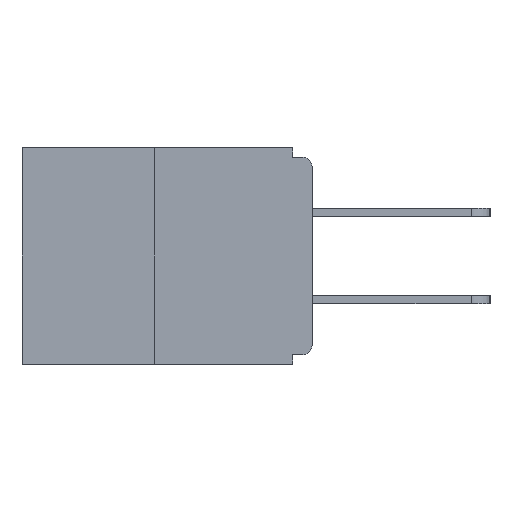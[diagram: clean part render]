
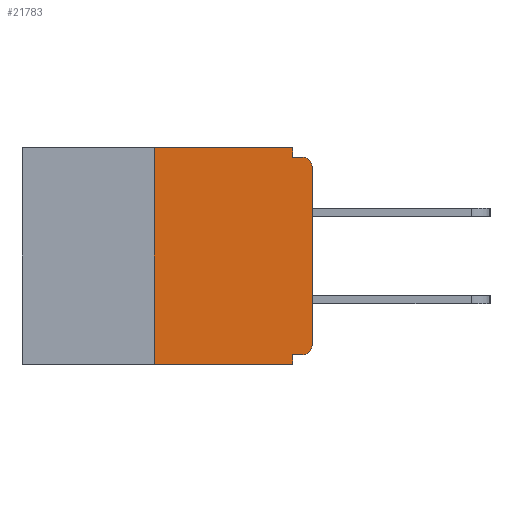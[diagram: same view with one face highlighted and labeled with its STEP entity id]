
A CAD part, left-side view. The second image highlights one B-rep face of the part: STEP entity #21783.
In plain terms, the highlighted planar face has unit normal (-1, 0, 0).
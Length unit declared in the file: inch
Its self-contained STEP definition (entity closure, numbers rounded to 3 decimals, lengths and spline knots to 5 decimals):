
#169 = EDGE_CURVE ( 'NONE', #12513, #19500, #6152, .T. ) ;
#231 = EDGE_CURVE ( 'NONE', #21958, #9194, #2474, .T. ) ;
#364 = DIRECTION ( 'NONE',  ( 0., 0., -1. ) ) ;
#468 = ORIENTED_EDGE ( 'NONE', *, *, #21047, .T. ) ;
#714 = EDGE_CURVE ( 'NONE', #6927, #9710, #7047, .T. ) ;
#760 = VERTEX_POINT ( 'NONE', #4860 ) ;
#1983 = VECTOR ( 'NONE', #9508, 39.37008 ) ;
#2123 = DIRECTION ( 'NONE',  ( 0., 1., 0. ) ) ;
#2136 = VECTOR ( 'NONE', #15917, 39.37008 ) ;
#2330 = EDGE_CURVE ( 'NONE', #12513, #8698, #7003, .T. ) ;
#2474 = LINE ( 'NONE', #5715, #12656 ) ;
#2747 = LINE ( 'NONE', #5709, #2136 ) ;
#3115 = LINE ( 'NONE', #14092, #24157 ) ;
#3269 = VECTOR ( 'NONE', #8938, 39.37008 ) ;
#3313 = PLANE ( 'NONE',  #25467 ) ;
#4295 = CARTESIAN_POINT ( 'NONE',  ( 0., 0.015, -0.03 ) ) ;
#4860 = CARTESIAN_POINT ( 'NONE',  ( 0., 0., -0.313 ) ) ;
#4899 = VECTOR ( 'NONE', #12804, 39.37008 ) ;
#5003 = ORIENTED_EDGE ( 'NONE', *, *, #16083, .T. ) ;
#5268 = CARTESIAN_POINT ( 'NONE',  ( 0., 0.015, -0.313 ) ) ;
#5463 = DIRECTION ( 'NONE',  ( 1., 0., 0. ) ) ;
#5709 = CARTESIAN_POINT ( 'NONE',  ( 0., 0., 0. ) ) ;
#5710 = ORIENTED_EDGE ( 'NONE', *, *, #19974, .T. ) ;
#5715 = CARTESIAN_POINT ( 'NONE',  ( 0., 0., -0.328 ) ) ;
#5799 = CARTESIAN_POINT ( 'NONE',  ( 0., 0.25, 0. ) ) ;
#5900 = ORIENTED_EDGE ( 'NONE', *, *, #2330, .T. ) ;
#6152 = LINE ( 'NONE', #5799, #16676 ) ;
#6377 = EDGE_CURVE ( 'NONE', #19500, #6927, #15220, .T. ) ;
#6667 = CARTESIAN_POINT ( 'NONE',  ( 0., 0.031, 0. ) ) ;
#6927 = VERTEX_POINT ( 'NONE', #13416 ) ;
#7003 = LINE ( 'NONE', #14622, #3269 ) ;
#7047 = LINE ( 'NONE', #6667, #4899 ) ;
#7219 = LINE ( 'NONE', #25058, #1983 ) ;
#8148 = VECTOR ( 'NONE', #19521, 39.37008 ) ;
#8647 = DIRECTION ( 'NONE',  ( 0., 0., -1. ) ) ;
#8698 = VERTEX_POINT ( 'NONE', #9263 ) ;
#8938 = DIRECTION ( 'NONE',  ( 0., -1., 0. ) ) ;
#9194 = VERTEX_POINT ( 'NONE', #22980 ) ;
#9197 = CARTESIAN_POINT ( 'NONE',  ( 0., 0., -0.03 ) ) ;
#9263 = CARTESIAN_POINT ( 'NONE',  ( 0., 0.031, -0.343 ) ) ;
#9508 = DIRECTION ( 'NONE',  ( 0., -1., 0. ) ) ;
#9710 = VERTEX_POINT ( 'NONE', #12374 ) ;
#10007 = DIRECTION ( 'NONE',  ( -1., 0., 0. ) ) ;
#10283 = ORIENTED_EDGE ( 'NONE', *, *, #24113, .F. ) ;
#10482 = AXIS2_PLACEMENT_3D ( 'NONE', #5268, #19121, #14927 ) ;
#10941 = EDGE_LOOP ( 'NONE', ( #18665, #18113, #5900, #25521, #11528, #5003, #468, #5710, #10283, #14709 ) ) ;
#11528 = ORIENTED_EDGE ( 'NONE', *, *, #231, .F. ) ;
#12374 = CARTESIAN_POINT ( 'NONE',  ( 0., 0.031, -0.015 ) ) ;
#12513 = VERTEX_POINT ( 'NONE', #19102 ) ;
#12656 = VECTOR ( 'NONE', #2123, 39.37008 ) ;
#12669 = CIRCLE ( 'NONE', #17830, 0.015 ) ;
#12804 = DIRECTION ( 'NONE',  ( 0., 0., -1. ) ) ;
#13416 = CARTESIAN_POINT ( 'NONE',  ( 0., 0.031, 0. ) ) ;
#13420 = DIRECTION ( 'NONE',  ( 0., 0., -1. ) ) ;
#13690 = DIRECTION ( 'NONE',  ( 0., 0., 1. ) ) ;
#13855 = CARTESIAN_POINT ( 'NONE',  ( 0., 0.015, -0.328 ) ) ;
#14092 = CARTESIAN_POINT ( 'NONE',  ( 0., 0.031, -0.343 ) ) ;
#14622 = CARTESIAN_POINT ( 'NONE',  ( 0., 0.46, -0.343 ) ) ;
#14709 = ORIENTED_EDGE ( 'NONE', *, *, #714, .F. ) ;
#14927 = DIRECTION ( 'NONE',  ( 0., 0., -1. ) ) ;
#15220 = LINE ( 'NONE', #15325, #8148 ) ;
#15325 = CARTESIAN_POINT ( 'NONE',  ( 0., 0.46, 0. ) ) ;
#15917 = DIRECTION ( 'NONE',  ( 0., 0., 1. ) ) ;
#16083 = EDGE_CURVE ( 'NONE', #21958, #760, #21189, .T. ) ;
#16676 = VECTOR ( 'NONE', #13690, 39.37008 ) ;
#17830 = AXIS2_PLACEMENT_3D ( 'NONE', #4295, #10007, #364 ) ;
#18070 = VERTEX_POINT ( 'NONE', #19401 ) ;
#18113 = ORIENTED_EDGE ( 'NONE', *, *, #169, .F. ) ;
#18665 = ORIENTED_EDGE ( 'NONE', *, *, #6377, .F. ) ;
#19102 = CARTESIAN_POINT ( 'NONE',  ( 0., 0.25, -0.343 ) ) ;
#19121 = DIRECTION ( 'NONE',  ( -1., 0., 0. ) ) ;
#19365 = EDGE_CURVE ( 'NONE', #9194, #8698, #3115, .T. ) ;
#19401 = CARTESIAN_POINT ( 'NONE',  ( 0., 0.015, -0.015 ) ) ;
#19500 = VERTEX_POINT ( 'NONE', #24193 ) ;
#19521 = DIRECTION ( 'NONE',  ( 0., -1., 0. ) ) ;
#19974 = EDGE_CURVE ( 'NONE', #23520, #18070, #12669, .T. ) ;
#21047 = EDGE_CURVE ( 'NONE', #760, #23520, #2747, .T. ) ;
#21189 = CIRCLE ( 'NONE', #10482, 0.015 ) ;
#21783 = ADVANCED_FACE ( 'NONE', ( #22188 ), #3313, .F. ) ;
#21958 = VERTEX_POINT ( 'NONE', #13855 ) ;
#22188 = FACE_OUTER_BOUND ( 'NONE', #10941, .T. ) ;
#22980 = CARTESIAN_POINT ( 'NONE',  ( 0., 0.031, -0.328 ) ) ;
#23520 = VERTEX_POINT ( 'NONE', #9197 ) ;
#24113 = EDGE_CURVE ( 'NONE', #9710, #18070, #7219, .T. ) ;
#24157 = VECTOR ( 'NONE', #8647, 39.37008 ) ;
#24193 = CARTESIAN_POINT ( 'NONE',  ( 0., 0.25, 0. ) ) ;
#25058 = CARTESIAN_POINT ( 'NONE',  ( 0., 0., -0.015 ) ) ;
#25340 = CARTESIAN_POINT ( 'NONE',  ( 0., 0.46, 0. ) ) ;
#25467 = AXIS2_PLACEMENT_3D ( 'NONE', #25340, #5463, #13420 ) ;
#25521 = ORIENTED_EDGE ( 'NONE', *, *, #19365, .F. ) ;
